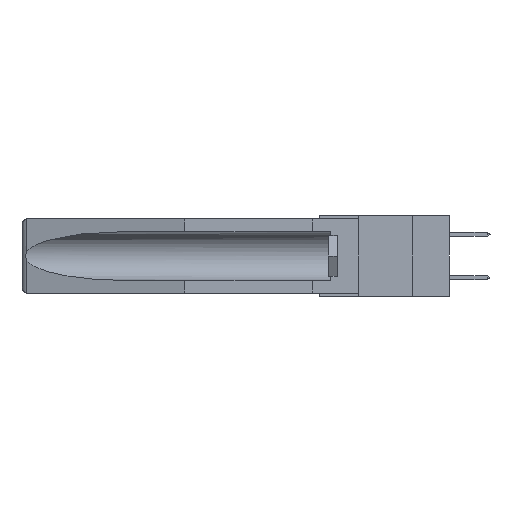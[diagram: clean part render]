
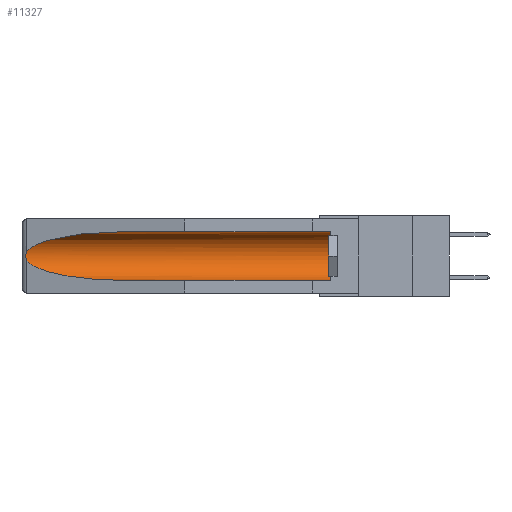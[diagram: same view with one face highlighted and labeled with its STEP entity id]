
A CAD part, left-side view. The second image highlights one B-rep face of the part: STEP entity #11327.
In plain terms, the highlighted cylindrical face has radius 2.857 mm (diameter 5.715 mm), a partial arc.
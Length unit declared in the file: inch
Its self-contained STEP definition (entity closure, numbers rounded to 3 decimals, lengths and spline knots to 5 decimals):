
#413 = ORIENTED_EDGE ( 'NONE', *, *, #1943, .T. ) ;
#765 = VERTEX_POINT ( 'NONE', #2124 ) ;
#1109 = DIRECTION ( 'NONE',  ( 0., 0., 1. ) ) ;
#1147 = CARTESIAN_POINT ( 'NONE',  ( 0.155, 0.126, -0.284 ) ) ;
#1253 = LINE ( 'NONE', #2219, #7780 ) ;
#1333 = CARTESIAN_POINT ( 'NONE',  ( 0.155, 0.126, -0.059 ) ) ;
#1442 = CARTESIAN_POINT ( 'NONE',  ( 0.26654, 1.53092, -0.15636 ) ) ;
#1604 = CARTESIAN_POINT ( 'NONE',  ( 0.155, -0.30754, -0.284 ) ) ;
#1663 = CARTESIAN_POINT ( 'NONE',  ( 0.26537, 1.52718, -0.14972 ) ) ;
#1943 = EDGE_CURVE ( 'NONE', #2562, #13548, #1253, .T. ) ;
#2123 = CARTESIAN_POINT ( 'NONE',  ( 0.25451, 1.48313, -0.24835 ) ) ;
#2124 = CARTESIAN_POINT ( 'NONE',  ( 0.155, 1.07973, -0.284 ) ) ;
#2219 = CARTESIAN_POINT ( 'NONE',  ( 0.155, -0.30754, -0.059 ) ) ;
#2467 = AXIS2_PLACEMENT_3D ( 'NONE', #15678, #9943, #7431 ) ;
#2505 = ORIENTED_EDGE ( 'NONE', *, *, #15679, .F. ) ;
#2562 = VERTEX_POINT ( 'NONE', #1333 ) ;
#2674 = CARTESIAN_POINT ( 'NONE',  ( 0.155, -0.30754, -0.1715 ) ) ;
#2704 = ORIENTED_EDGE ( 'NONE', *, *, #4636, .T. ) ;
#2945 = DIRECTION ( 'NONE',  ( 0., 1., 0. ) ) ;
#3027 = CARTESIAN_POINT ( 'NONE',  ( 0.26597, 1.52961, -0.15275 ) ) ;
#3334 = CARTESIAN_POINT ( 'NONE',  ( 0.25451, 1.48313, -0.09465 ) ) ;
#3583 = CARTESIAN_POINT ( 'NONE',  ( 0.21114, 1.30732, -0.284 ) ) ;
#3760 = CARTESIAN_POINT ( 'NONE',  ( 0.26537, 1.52718, -0.19328 ) ) ;
#3820 =( BOUNDED_CURVE ( )  B_SPLINE_CURVE ( 3, ( #3760, #2123, #3583, #4957 ),
 .UNSPECIFIED., .F., .F. ) 
 B_SPLINE_CURVE_WITH_KNOTS ( ( 4, 4 ),
 ( 0.1948, 1.5708 ),
 .UNSPECIFIED. ) 
 CURVE ( )  GEOMETRIC_REPRESENTATION_ITEM ( )  RATIONAL_B_SPLINE_CURVE ( ( 1., 0.848, 0.848, 1. ) ) 
 REPRESENTATION_ITEM ( '' )  );
#4169 = CARTESIAN_POINT ( 'NONE',  ( 0.26597, 1.5296, -0.19026 ) ) ;
#4413 = EDGE_LOOP ( 'NONE', ( #7721, #2704, #11865, #2505, #15931, #413 ) ) ;
#4636 = EDGE_CURVE ( 'NONE', #15013, #11908, #5492, .T. ) ;
#4734 = CIRCLE ( 'NONE', #2467, 0.1125 ) ;
#4957 = CARTESIAN_POINT ( 'NONE',  ( 0.155, 1.07973, -0.284 ) ) ;
#5377 = DIRECTION ( 'NONE',  ( 0., 1., 0. ) ) ;
#5492 = B_SPLINE_CURVE_WITH_KNOTS ( 'NONE', 3,
 ( #12518, #3027, #1442, #8410, #5801, #16695, #11042, #12407, #4169, #13785 ),
 .UNSPECIFIED., .F., .F.,
 ( 4, 2, 2, 2, 4 ),
 ( 0., 0.00029, 0.00058, 0.00087, 0.00117 ),
 .UNSPECIFIED. ) ;
#5785 = CYLINDRICAL_SURFACE ( 'NONE', #13430, 0.1125 ) ;
#5801 = CARTESIAN_POINT ( 'NONE',  ( 0.2675, 1.53308, -0.16763 ) ) ;
#6514 = VECTOR ( 'NONE', #2945, 39.37008 ) ;
#7431 = DIRECTION ( 'NONE',  ( 0., 0., 1. ) ) ;
#7545 = CARTESIAN_POINT ( 'NONE',  ( 0.155, 1.07973, -0.059 ) ) ;
#7721 = ORIENTED_EDGE ( 'NONE', *, *, #8959, .T. ) ;
#7780 = VECTOR ( 'NONE', #10563, 39.37008 ) ;
#8410 = CARTESIAN_POINT ( 'NONE',  ( 0.2673, 1.5327, -0.16383 ) ) ;
#8529 = CARTESIAN_POINT ( 'NONE',  ( 0.21114, 1.30732, -0.059 ) ) ;
#8959 = EDGE_CURVE ( 'NONE', #13548, #15013, #13193, .T. ) ;
#9663 = CARTESIAN_POINT ( 'NONE',  ( 0.26537, 1.52718, -0.19328 ) ) ;
#9844 = CARTESIAN_POINT ( 'NONE',  ( 0.155, 1.07973, -0.059 ) ) ;
#9943 = DIRECTION ( 'NONE',  ( 0., -1., 0. ) ) ;
#10563 = DIRECTION ( 'NONE',  ( 0., 1., 0. ) ) ;
#11042 = CARTESIAN_POINT ( 'NONE',  ( 0.2673, 1.53269, -0.17917 ) ) ;
#11327 = ADVANCED_FACE ( 'NONE', ( #17629 ), #5785, .F. ) ;
#11865 = ORIENTED_EDGE ( 'NONE', *, *, #13638, .T. ) ;
#11908 = VERTEX_POINT ( 'NONE', #9663 ) ;
#12407 = CARTESIAN_POINT ( 'NONE',  ( 0.26655, 1.53094, -0.18657 ) ) ;
#12518 = CARTESIAN_POINT ( 'NONE',  ( 0.26537, 1.52718, -0.14972 ) ) ;
#13193 =( BOUNDED_CURVE ( )  B_SPLINE_CURVE ( 3, ( #9844, #8529, #3334, #16287 ),
 .UNSPECIFIED., .F., .F. ) 
 B_SPLINE_CURVE_WITH_KNOTS ( ( 4, 4 ),
 ( 4.71239, 6.08839 ),
 .UNSPECIFIED. ) 
 CURVE ( )  GEOMETRIC_REPRESENTATION_ITEM ( )  RATIONAL_B_SPLINE_CURVE ( ( 1., 0.848, 0.848, 1. ) ) 
 REPRESENTATION_ITEM ( '' )  );
#13430 = AXIS2_PLACEMENT_3D ( 'NONE', #2674, #5377, #1109 ) ;
#13548 = VERTEX_POINT ( 'NONE', #7545 ) ;
#13638 = EDGE_CURVE ( 'NONE', #11908, #765, #3820, .T. ) ;
#13785 = CARTESIAN_POINT ( 'NONE',  ( 0.26537, 1.52718, -0.19328 ) ) ;
#15013 = VERTEX_POINT ( 'NONE', #1663 ) ;
#15678 = CARTESIAN_POINT ( 'NONE',  ( 0.155, 0.126, -0.1715 ) ) ;
#15679 = EDGE_CURVE ( 'NONE', #16048, #765, #16843, .T. ) ;
#15931 = ORIENTED_EDGE ( 'NONE', *, *, #17675, .T. ) ;
#16048 = VERTEX_POINT ( 'NONE', #1147 ) ;
#16287 = CARTESIAN_POINT ( 'NONE',  ( 0.26537, 1.52718, -0.14972 ) ) ;
#16695 = CARTESIAN_POINT ( 'NONE',  ( 0.2675, 1.53308, -0.17534 ) ) ;
#16843 = LINE ( 'NONE', #1604, #6514 ) ;
#17629 = FACE_OUTER_BOUND ( 'NONE', #4413, .T. ) ;
#17675 = EDGE_CURVE ( 'NONE', #16048, #2562, #4734, .T. ) ;
